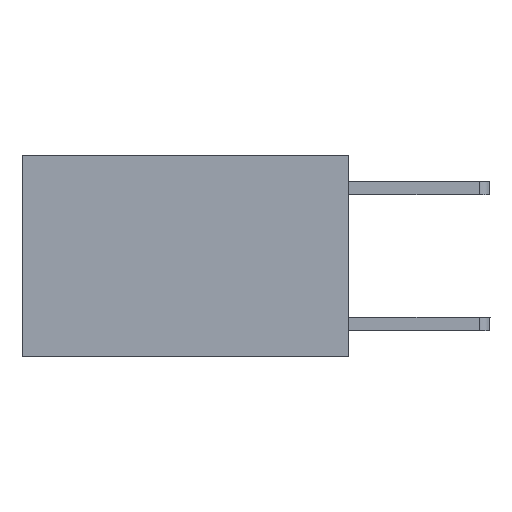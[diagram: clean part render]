
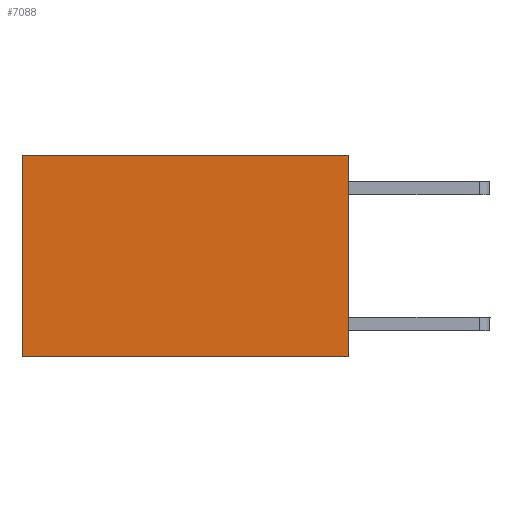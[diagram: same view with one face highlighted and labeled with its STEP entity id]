
A CAD part, left-side view. The second image highlights one B-rep face of the part: STEP entity #7088.
In plain terms, the highlighted planar face has unit normal (-1, 0, 0).
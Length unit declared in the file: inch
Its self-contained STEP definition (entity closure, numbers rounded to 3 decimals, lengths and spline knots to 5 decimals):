
#562 = CARTESIAN_POINT ( 'NONE',  ( 0.2625, 0.6, 0. ) ) ;
#1069 = VERTEX_POINT ( 'NONE', #5172 ) ;
#1155 = VECTOR ( 'NONE', #7957, 39.37008 ) ;
#1303 = LINE ( 'NONE', #7849, #1155 ) ;
#1522 = EDGE_CURVE ( 'NONE', #7925, #9552, #6125, .T. ) ;
#1591 = CARTESIAN_POINT ( 'NONE',  ( 0.2625, 0., 0. ) ) ;
#2042 = DIRECTION ( 'NONE',  ( 0., 0., -1. ) ) ;
#2679 = AXIS2_PLACEMENT_3D ( 'NONE', #5530, #7300, #2042 ) ;
#3016 = EDGE_CURVE ( 'NONE', #7925, #10790, #1303, .T. ) ;
#3051 = FACE_OUTER_BOUND ( 'NONE', #10166, .T. ) ;
#3299 = VECTOR ( 'NONE', #9184, 39.37008 ) ;
#3369 = ORIENTED_EDGE ( 'NONE', *, *, #9152, .F. ) ;
#3566 = ORIENTED_EDGE ( 'NONE', *, *, #1522, .T. ) ;
#4096 = DIRECTION ( 'NONE',  ( 0., 1., 0. ) ) ;
#4450 = VECTOR ( 'NONE', #7583, 39.37008 ) ;
#4995 = ORIENTED_EDGE ( 'NONE', *, *, #3016, .F. ) ;
#5172 = CARTESIAN_POINT ( 'NONE',  ( 0.2625, 0.6, -0.37 ) ) ;
#5530 = CARTESIAN_POINT ( 'NONE',  ( 0.2625, 0., 0. ) ) ;
#5638 = LINE ( 'NONE', #10009, #3299 ) ;
#5838 = EDGE_CURVE ( 'NONE', #9552, #1069, #9096, .T. ) ;
#6065 = VECTOR ( 'NONE', #4096, 39.37008 ) ;
#6125 = LINE ( 'NONE', #1591, #6065 ) ;
#6414 = PLANE ( 'NONE',  #2679 ) ;
#7088 = ADVANCED_FACE ( 'NONE', ( #3051 ), #6414, .F. ) ;
#7212 = CARTESIAN_POINT ( 'NONE',  ( 0.2625, 0.6, 0. ) ) ;
#7214 = ORIENTED_EDGE ( 'NONE', *, *, #5838, .T. ) ;
#7300 = DIRECTION ( 'NONE',  ( 1., 0., 0. ) ) ;
#7583 = DIRECTION ( 'NONE',  ( 0., 0., -1. ) ) ;
#7849 = CARTESIAN_POINT ( 'NONE',  ( 0.2625, 0., 0. ) ) ;
#7925 = VERTEX_POINT ( 'NONE', #8573 ) ;
#7957 = DIRECTION ( 'NONE',  ( 0., 0., -1. ) ) ;
#8573 = CARTESIAN_POINT ( 'NONE',  ( 0.2625, 0., 0. ) ) ;
#9096 = LINE ( 'NONE', #562, #4450 ) ;
#9152 = EDGE_CURVE ( 'NONE', #10790, #1069, #5638, .T. ) ;
#9184 = DIRECTION ( 'NONE',  ( 0., 1., 0. ) ) ;
#9552 = VERTEX_POINT ( 'NONE', #7212 ) ;
#10009 = CARTESIAN_POINT ( 'NONE',  ( 0.2625, 0., -0.37 ) ) ;
#10166 = EDGE_LOOP ( 'NONE', ( #7214, #3369, #4995, #3566 ) ) ;
#10790 = VERTEX_POINT ( 'NONE', #11022 ) ;
#11022 = CARTESIAN_POINT ( 'NONE',  ( 0.2625, 0., -0.37 ) ) ;
